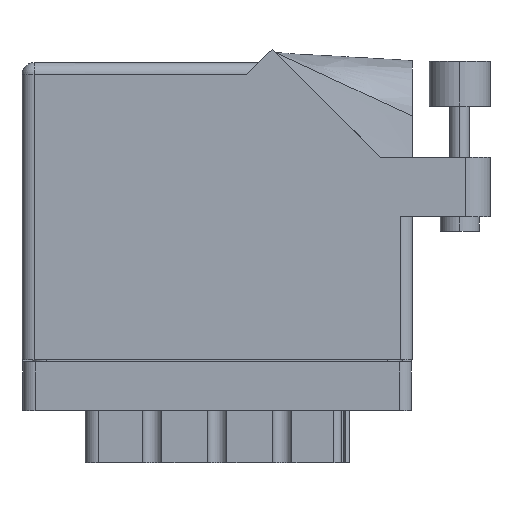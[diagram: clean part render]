
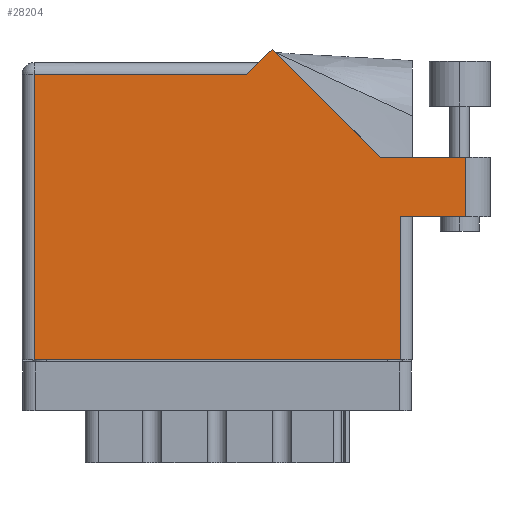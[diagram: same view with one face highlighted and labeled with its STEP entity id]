
A CAD part, front view. The second image highlights one B-rep face of the part: STEP entity #28204.
In plain terms, the highlighted face is planar.
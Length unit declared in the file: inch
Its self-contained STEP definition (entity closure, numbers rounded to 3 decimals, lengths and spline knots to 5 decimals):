
#634 = LINE ( 'NONE', #5009, #23469 ) ;
#2505 = DIRECTION ( 'NONE',  ( 0., 0., -1. ) ) ;
#2650 = DIRECTION ( 'NONE',  ( -1., 0., 0. ) ) ;
#2875 = VERTEX_POINT ( 'NONE', #27602 ) ;
#3478 = VERTEX_POINT ( 'NONE', #7799 ) ;
#4493 = LINE ( 'NONE', #29015, #25344 ) ;
#5009 = CARTESIAN_POINT ( 'NONE',  ( 0., 0., 0. ) ) ;
#5327 = DIRECTION ( 'NONE',  ( 1., 0., 0. ) ) ;
#6250 = AXIS2_PLACEMENT_3D ( 'NONE', #37294, #2505, #2650 ) ;
#6435 = EDGE_CURVE ( 'NONE', #3478, #6933, #19912, .T. ) ;
#6584 = ORIENTED_EDGE ( 'NONE', *, *, #39442, .T. ) ;
#6933 = VERTEX_POINT ( 'NONE', #30289 ) ;
#7377 = CARTESIAN_POINT ( 'NONE',  ( 0.062, 1.468, 0. ) ) ;
#7799 = CARTESIAN_POINT ( 'NONE',  ( 2.285, 0.737, 0. ) ) ;
#7942 = DIRECTION ( 'NONE',  ( -0.707, 0.707, 0. ) ) ;
#8272 = ORIENTED_EDGE ( 'NONE', *, *, #10475, .T. ) ;
#8927 = CARTESIAN_POINT ( 'NONE',  ( 1.155, 1.468, 0. ) ) ;
#10475 = EDGE_CURVE ( 'NONE', #27793, #2875, #32192, .T. ) ;
#10981 = ORIENTED_EDGE ( 'NONE', *, *, #31493, .T. ) ;
#12264 = DIRECTION ( 'NONE',  ( -1., 0., 0. ) ) ;
#12408 = CARTESIAN_POINT ( 'NONE',  ( 0., 1.468, 0. ) ) ;
#12627 = EDGE_CURVE ( 'NONE', #2875, #26492, #19970, .T. ) ;
#13277 = ORIENTED_EDGE ( 'NONE', *, *, #14061, .T. ) ;
#13590 = LINE ( 'NONE', #12408, #35569 ) ;
#14061 = EDGE_CURVE ( 'NONE', #6933, #27793, #4493, .T. ) ;
#14788 = CARTESIAN_POINT ( 'NONE',  ( 1.948, 0., 0. ) ) ;
#15906 = LINE ( 'NONE', #37756, #29406 ) ;
#16627 = CARTESIAN_POINT ( 'NONE',  ( 1.84442, 1.044, 0. ) ) ;
#16659 = VECTOR ( 'NONE', #7942, 39.37008 ) ;
#17681 = ORIENTED_EDGE ( 'NONE', *, *, #6435, .T. ) ;
#17833 = ORIENTED_EDGE ( 'NONE', *, *, #21584, .T. ) ;
#17913 = CARTESIAN_POINT ( 'NONE',  ( 0.062, 0., 0. ) ) ;
#18235 = CARTESIAN_POINT ( 'NONE',  ( 1.217, 1.53, 0. ) ) ;
#18400 = VECTOR ( 'NONE', #40231, 39.37008 ) ;
#19011 = VERTEX_POINT ( 'NONE', #34038 ) ;
#19760 = DIRECTION ( 'NONE',  ( -1., 0., 0. ) ) ;
#19912 = LINE ( 'NONE', #27802, #18400 ) ;
#19970 = LINE ( 'NONE', #18235, #31490 ) ;
#20279 = LINE ( 'NONE', #17913, #27790 ) ;
#21432 = DIRECTION ( 'NONE',  ( -0.707, -0.707, 0. ) ) ;
#21584 = EDGE_CURVE ( 'NONE', #26492, #38456, #13590, .T. ) ;
#22093 = VECTOR ( 'NONE', #33991, 39.37008 ) ;
#23271 = FACE_OUTER_BOUND ( 'NONE', #38417, .T. ) ;
#23469 = VECTOR ( 'NONE', #5327, 39.37008 ) ;
#23568 = ORIENTED_EDGE ( 'NONE', *, *, #12627, .T. ) ;
#24455 = EDGE_CURVE ( 'NONE', #19011, #3478, #39552, .T. ) ;
#25344 = VECTOR ( 'NONE', #19760, 39.37008 ) ;
#26273 = ORIENTED_EDGE ( 'NONE', *, *, #27567, .T. ) ;
#26492 = VERTEX_POINT ( 'NONE', #8927 ) ;
#26944 = CARTESIAN_POINT ( 'NONE',  ( 1.84442, 1.044, 0. ) ) ;
#27567 = EDGE_CURVE ( 'NONE', #38456, #37573, #20279, .T. ) ;
#27602 = CARTESIAN_POINT ( 'NONE',  ( 1.28771, 1.60071, 0. ) ) ;
#27790 = VECTOR ( 'NONE', #36897, 39.37008 ) ;
#27793 = VERTEX_POINT ( 'NONE', #16627 ) ;
#27802 = CARTESIAN_POINT ( 'NONE',  ( 2.285, 1.044, 0. ) ) ;
#28204 = ADVANCED_FACE ( 'NONE', ( #23271 ), #40889, .F. ) ;
#29015 = CARTESIAN_POINT ( 'NONE',  ( 2.41, 1.044, 0. ) ) ;
#29406 = VECTOR ( 'NONE', #37623, 39.37008 ) ;
#30289 = CARTESIAN_POINT ( 'NONE',  ( 2.285, 1.044, 0. ) ) ;
#31490 = VECTOR ( 'NONE', #21432, 39.37008 ) ;
#31493 = EDGE_CURVE ( 'NONE', #37573, #37284, #634, .T. ) ;
#32192 = LINE ( 'NONE', #26944, #16659 ) ;
#33991 = DIRECTION ( 'NONE',  ( 1., 0., 0. ) ) ;
#34038 = CARTESIAN_POINT ( 'NONE',  ( 1.948, 0.737, 0. ) ) ;
#35569 = VECTOR ( 'NONE', #12264, 39.37008 ) ;
#36897 = DIRECTION ( 'NONE',  ( 0., -1., 0. ) ) ;
#37284 = VERTEX_POINT ( 'NONE', #14788 ) ;
#37294 = CARTESIAN_POINT ( 'NONE',  ( 0., 1.53, 0. ) ) ;
#37354 = CARTESIAN_POINT ( 'NONE',  ( 0.062, 0., 0. ) ) ;
#37573 = VERTEX_POINT ( 'NONE', #37354 ) ;
#37623 = DIRECTION ( 'NONE',  ( 0., 1., 0. ) ) ;
#37756 = CARTESIAN_POINT ( 'NONE',  ( 1.948, 0.737, 0. ) ) ;
#37933 = ORIENTED_EDGE ( 'NONE', *, *, #24455, .T. ) ;
#38417 = EDGE_LOOP ( 'NONE', ( #37933, #17681, #13277, #8272, #23568, #17833, #26273, #10981, #6584 ) ) ;
#38456 = VERTEX_POINT ( 'NONE', #7377 ) ;
#39442 = EDGE_CURVE ( 'NONE', #37284, #19011, #15906, .T. ) ;
#39552 = LINE ( 'NONE', #40382, #22093 ) ;
#40231 = DIRECTION ( 'NONE',  ( 0., 1., 0. ) ) ;
#40382 = CARTESIAN_POINT ( 'NONE',  ( 2.01, 0.737, 0. ) ) ;
#40889 = PLANE ( 'NONE',  #6250 ) ;
